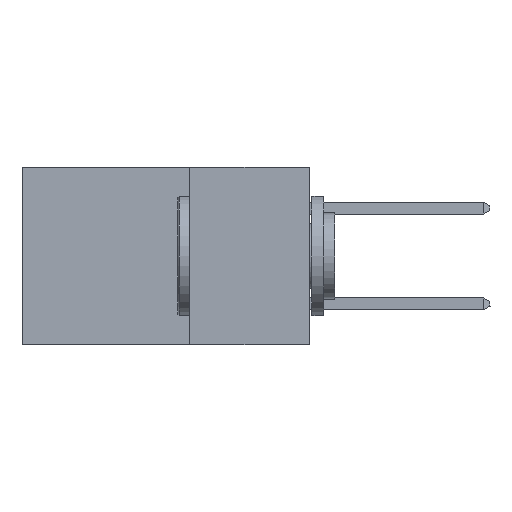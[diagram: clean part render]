
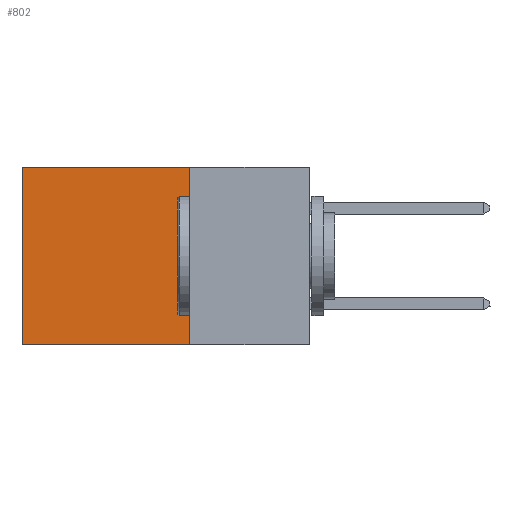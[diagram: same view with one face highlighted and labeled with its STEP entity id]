
A CAD part, left-side view. The second image highlights one B-rep face of the part: STEP entity #802.
In plain terms, the highlighted planar face has unit normal (-1, 0, 0).
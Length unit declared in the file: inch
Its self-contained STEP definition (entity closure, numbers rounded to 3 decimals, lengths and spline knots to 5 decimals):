
#148 = EDGE_CURVE ( 'NONE', #938, #17648, #12557, .T. ) ;
#230 = CARTESIAN_POINT ( 'NONE',  ( 0.2875, 0.25, -0.37 ) ) ;
#802 = ADVANCED_FACE ( 'NONE', ( #16702 ), #13237, .F. ) ;
#938 = VERTEX_POINT ( 'NONE', #1092 ) ;
#1052 = CARTESIAN_POINT ( 'NONE',  ( 0.2875, 0.6, 0. ) ) ;
#1092 = CARTESIAN_POINT ( 'NONE',  ( 0.2875, 0.25, 0. ) ) ;
#1224 = CARTESIAN_POINT ( 'NONE',  ( 0.2875, 0.25, -0.37 ) ) ;
#1875 = VECTOR ( 'NONE', #15833, 39.37008 ) ;
#1983 = CARTESIAN_POINT ( 'NONE',  ( 0.2875, 0.6, -0.37 ) ) ;
#2021 = DIRECTION ( 'NONE',  ( 0., 1., 0. ) ) ;
#3935 = ORIENTED_EDGE ( 'NONE', *, *, #10946, .T. ) ;
#5960 = ORIENTED_EDGE ( 'NONE', *, *, #25978, .F. ) ;
#7287 = ORIENTED_EDGE ( 'NONE', *, *, #11982, .T. ) ;
#9007 = DIRECTION ( 'NONE',  ( 0., 0., -1. ) ) ;
#9796 = VECTOR ( 'NONE', #9007, 39.37008 ) ;
#10239 = CARTESIAN_POINT ( 'NONE',  ( 0.2875, 0.25, 0. ) ) ;
#10441 = EDGE_LOOP ( 'NONE', ( #3935, #5960, #24426, #7287 ) ) ;
#10703 = VECTOR ( 'NONE', #2021, 39.37008 ) ;
#10946 = EDGE_CURVE ( 'NONE', #13888, #26786, #20898, .T. ) ;
#11357 = LINE ( 'NONE', #1224, #1875 ) ;
#11982 = EDGE_CURVE ( 'NONE', #938, #13888, #18210, .T. ) ;
#12557 = LINE ( 'NONE', #12943, #18419 ) ;
#12943 = CARTESIAN_POINT ( 'NONE',  ( 0.2875, 0.25, 0. ) ) ;
#13158 = DIRECTION ( 'NONE',  ( 0., 0., -1. ) ) ;
#13237 = PLANE ( 'NONE',  #15046 ) ;
#13888 = VERTEX_POINT ( 'NONE', #19031 ) ;
#15046 = AXIS2_PLACEMENT_3D ( 'NONE', #21640, #15249, #13158 ) ;
#15249 = DIRECTION ( 'NONE',  ( 1., 0., 0. ) ) ;
#15833 = DIRECTION ( 'NONE',  ( 0., 1., 0. ) ) ;
#16702 = FACE_OUTER_BOUND ( 'NONE', #10441, .T. ) ;
#17648 = VERTEX_POINT ( 'NONE', #230 ) ;
#18210 = LINE ( 'NONE', #10239, #10703 ) ;
#18419 = VECTOR ( 'NONE', #24147, 39.37008 ) ;
#19031 = CARTESIAN_POINT ( 'NONE',  ( 0.2875, 0.6, 0. ) ) ;
#20898 = LINE ( 'NONE', #1052, #9796 ) ;
#21640 = CARTESIAN_POINT ( 'NONE',  ( 0.2875, 0.25, 0. ) ) ;
#24147 = DIRECTION ( 'NONE',  ( 0., 0., -1. ) ) ;
#24426 = ORIENTED_EDGE ( 'NONE', *, *, #148, .F. ) ;
#25978 = EDGE_CURVE ( 'NONE', #17648, #26786, #11357, .T. ) ;
#26786 = VERTEX_POINT ( 'NONE', #1983 ) ;
